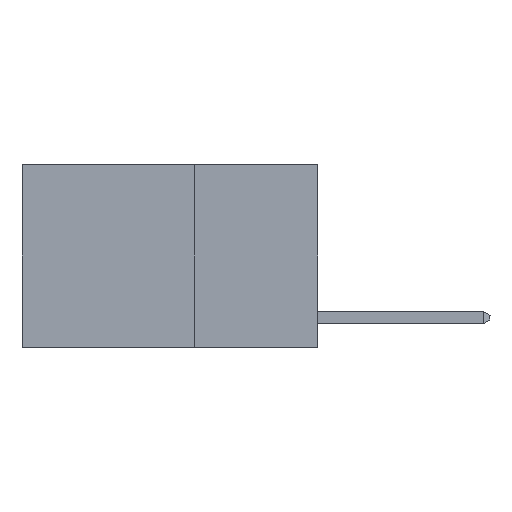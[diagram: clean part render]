
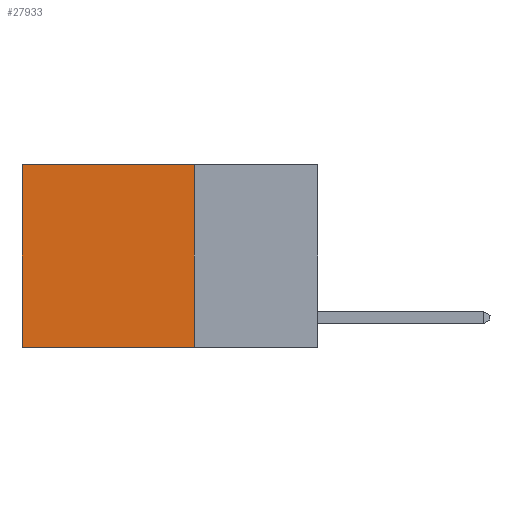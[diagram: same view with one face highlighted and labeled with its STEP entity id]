
A CAD part, left-side view. The second image highlights one B-rep face of the part: STEP entity #27933.
In plain terms, the highlighted planar face has unit normal (-1, 0, 0).
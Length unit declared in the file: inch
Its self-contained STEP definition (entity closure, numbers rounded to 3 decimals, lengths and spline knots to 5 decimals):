
#1082 = EDGE_CURVE ( 'NONE', #10682, #6711, #14480, .T. ) ;
#2484 = DIRECTION ( 'NONE',  ( 0., 1., 0. ) ) ;
#3732 = VERTEX_POINT ( 'NONE', #5527 ) ;
#4274 = ORIENTED_EDGE ( 'NONE', *, *, #20694, .F. ) ;
#4339 = CARTESIAN_POINT ( 'NONE',  ( 0.2625, 0.25, 0. ) ) ;
#4561 = CARTESIAN_POINT ( 'NONE',  ( 0.2625, 0.25, 0. ) ) ;
#5527 = CARTESIAN_POINT ( 'NONE',  ( 0.2625, 0.25, 0. ) ) ;
#6711 = VERTEX_POINT ( 'NONE', #17780 ) ;
#6826 = FACE_OUTER_BOUND ( 'NONE', #20236, .T. ) ;
#6870 = PLANE ( 'NONE',  #27062 ) ;
#7657 = VERTEX_POINT ( 'NONE', #12361 ) ;
#9098 = VECTOR ( 'NONE', #25306, 39.37008 ) ;
#9208 = ORIENTED_EDGE ( 'NONE', *, *, #1082, .T. ) ;
#9393 = CARTESIAN_POINT ( 'NONE',  ( 0.2625, 0.6, 0. ) ) ;
#10682 = VERTEX_POINT ( 'NONE', #23675 ) ;
#11472 = DIRECTION ( 'NONE',  ( 0., 0., -1. ) ) ;
#12361 = CARTESIAN_POINT ( 'NONE',  ( 0.2625, 0.25, -0.37 ) ) ;
#12585 = VECTOR ( 'NONE', #27536, 39.37008 ) ;
#13729 = LINE ( 'NONE', #18572, #19130 ) ;
#14480 = LINE ( 'NONE', #9393, #9098 ) ;
#15969 = VECTOR ( 'NONE', #29320, 39.37008 ) ;
#17160 = ORIENTED_EDGE ( 'NONE', *, *, #18259, .F. ) ;
#17607 = EDGE_CURVE ( 'NONE', #3732, #10682, #13729, .T. ) ;
#17780 = CARTESIAN_POINT ( 'NONE',  ( 0.2625, 0.6, -0.37 ) ) ;
#18259 = EDGE_CURVE ( 'NONE', #7657, #6711, #24684, .T. ) ;
#18572 = CARTESIAN_POINT ( 'NONE',  ( 0.2625, 0.25, 0. ) ) ;
#19130 = VECTOR ( 'NONE', #2484, 39.37008 ) ;
#20236 = EDGE_LOOP ( 'NONE', ( #9208, #17160, #4274, #20322 ) ) ;
#20322 = ORIENTED_EDGE ( 'NONE', *, *, #17607, .T. ) ;
#20694 = EDGE_CURVE ( 'NONE', #3732, #7657, #22004, .T. ) ;
#22004 = LINE ( 'NONE', #4339, #15969 ) ;
#23675 = CARTESIAN_POINT ( 'NONE',  ( 0.2625, 0.6, 0. ) ) ;
#24684 = LINE ( 'NONE', #25295, #12585 ) ;
#25081 = DIRECTION ( 'NONE',  ( 1., 0., 0. ) ) ;
#25295 = CARTESIAN_POINT ( 'NONE',  ( 0.2625, 0.25, -0.37 ) ) ;
#25306 = DIRECTION ( 'NONE',  ( 0., 0., -1. ) ) ;
#27062 = AXIS2_PLACEMENT_3D ( 'NONE', #4561, #25081, #11472 ) ;
#27536 = DIRECTION ( 'NONE',  ( 0., 1., 0. ) ) ;
#27933 = ADVANCED_FACE ( 'NONE', ( #6826 ), #6870, .F. ) ;
#29320 = DIRECTION ( 'NONE',  ( 0., 0., -1. ) ) ;
